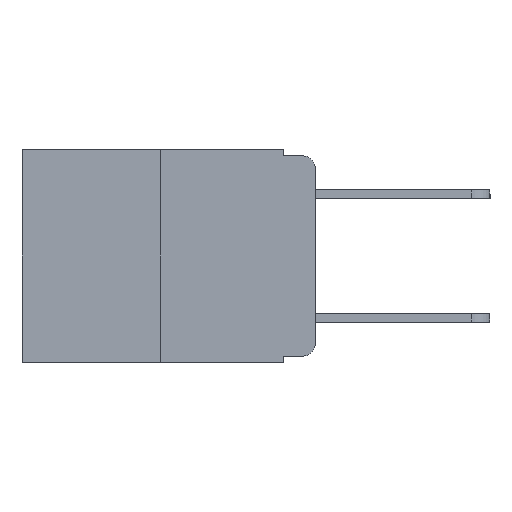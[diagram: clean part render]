
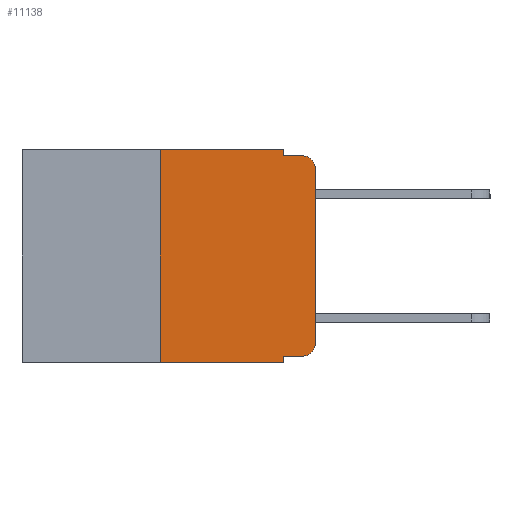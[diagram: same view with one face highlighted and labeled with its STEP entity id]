
A CAD part, left-side view. The second image highlights one B-rep face of the part: STEP entity #11138.
In plain terms, the highlighted planar face has unit normal (-1, 0, 0).
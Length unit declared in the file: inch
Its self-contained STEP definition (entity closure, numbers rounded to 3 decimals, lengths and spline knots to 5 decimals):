
#94 = VERTEX_POINT ( 'NONE', #11074 ) ;
#110 = DIRECTION ( 'NONE',  ( 0., 0., -1. ) ) ;
#378 = LINE ( 'NONE', #8288, #10097 ) ;
#680 = EDGE_CURVE ( 'NONE', #3848, #2437, #4072, .T. ) ;
#988 = VERTEX_POINT ( 'NONE', #6801 ) ;
#1204 = DIRECTION ( 'NONE',  ( 0., -1., 0. ) ) ;
#1396 = LINE ( 'NONE', #10054, #5968 ) ;
#1401 = ORIENTED_EDGE ( 'NONE', *, *, #8843, .F. ) ;
#1557 = VECTOR ( 'NONE', #3485, 39.37008 ) ;
#1706 = CARTESIAN_POINT ( 'NONE',  ( 0., 0.051, 0. ) ) ;
#1749 = ORIENTED_EDGE ( 'NONE', *, *, #1933, .F. ) ;
#1764 = CARTESIAN_POINT ( 'NONE',  ( 0., 0.473, -0.343 ) ) ;
#1769 = CARTESIAN_POINT ( 'NONE',  ( 0., 0.051, 0. ) ) ;
#1846 = EDGE_CURVE ( 'NONE', #5021, #2993, #1396, .T. ) ;
#1866 = EDGE_CURVE ( 'NONE', #2993, #94, #3632, .T. ) ;
#1905 = EDGE_CURVE ( 'NONE', #988, #94, #9902, .T. ) ;
#1933 = EDGE_CURVE ( 'NONE', #4409, #988, #5375, .T. ) ;
#1965 = EDGE_CURVE ( 'NONE', #3848, #10779, #9175, .T. ) ;
#1985 = EDGE_CURVE ( 'NONE', #4274, #2437, #4609, .T. ) ;
#2002 = EDGE_CURVE ( 'NONE', #4274, #9136, #6937, .T. ) ;
#2294 = CARTESIAN_POINT ( 'NONE',  ( 0., 0.473, 0. ) ) ;
#2395 = CARTESIAN_POINT ( 'NONE',  ( 0., 0.02, -0.333 ) ) ;
#2409 = CARTESIAN_POINT ( 'NONE',  ( 0., 0., -0.03 ) ) ;
#2437 = VERTEX_POINT ( 'NONE', #11195 ) ;
#2537 = EDGE_CURVE ( 'NONE', #9136, #5021, #9658, .T. ) ;
#2837 = DIRECTION ( 'NONE',  ( 0., -1., 0. ) ) ;
#2993 = VERTEX_POINT ( 'NONE', #2409 ) ;
#3011 = ORIENTED_EDGE ( 'NONE', *, *, #1866, .T. ) ;
#3067 = CARTESIAN_POINT ( 'NONE',  ( 0., 0.051, 0. ) ) ;
#3081 = ORIENTED_EDGE ( 'NONE', *, *, #1846, .T. ) ;
#3084 = VECTOR ( 'NONE', #1204, 39.37008 ) ;
#3246 = DIRECTION ( 'NONE',  ( 0., 0., -1. ) ) ;
#3353 = ORIENTED_EDGE ( 'NONE', *, *, #2537, .T. ) ;
#3485 = DIRECTION ( 'NONE',  ( 0., -1., 0. ) ) ;
#3632 = CIRCLE ( 'NONE', #4986, 0.02 ) ;
#3761 = AXIS2_PLACEMENT_3D ( 'NONE', #9645, #9270, #9260 ) ;
#3848 = VERTEX_POINT ( 'NONE', #4613 ) ;
#4072 = LINE ( 'NONE', #1764, #1557 ) ;
#4073 = CARTESIAN_POINT ( 'NONE',  ( 0., 0., -0.313 ) ) ;
#4075 = CARTESIAN_POINT ( 'NONE',  ( 0., 0.051, -0.333 ) ) ;
#4274 = VERTEX_POINT ( 'NONE', #9355 ) ;
#4409 = VERTEX_POINT ( 'NONE', #1706 ) ;
#4609 = LINE ( 'NONE', #3067, #8918 ) ;
#4613 = CARTESIAN_POINT ( 'NONE',  ( 0., 0.25, -0.343 ) ) ;
#4986 = AXIS2_PLACEMENT_3D ( 'NONE', #8393, #6985, #7596 ) ;
#5021 = VERTEX_POINT ( 'NONE', #4073 ) ;
#5117 = VECTOR ( 'NONE', #110, 39.37008 ) ;
#5198 = ORIENTED_EDGE ( 'NONE', *, *, #680, .T. ) ;
#5299 = ORIENTED_EDGE ( 'NONE', *, *, #2002, .T. ) ;
#5375 = LINE ( 'NONE', #1769, #5117 ) ;
#5539 = DIRECTION ( 'NONE',  ( 0., -1., 0. ) ) ;
#5758 = ORIENTED_EDGE ( 'NONE', *, *, #1905, .F. ) ;
#5968 = VECTOR ( 'NONE', #10854, 39.37008 ) ;
#6409 = DIRECTION ( 'NONE',  ( 0., 0., 1. ) ) ;
#6436 = EDGE_LOOP ( 'NONE', ( #3081, #3011, #5758, #1749, #1401, #10562, #5198, #8328, #5299, #3353 ) ) ;
#6668 = VECTOR ( 'NONE', #2837, 39.37008 ) ;
#6801 = CARTESIAN_POINT ( 'NONE',  ( 0., 0.051, -0.01 ) ) ;
#6937 = LINE ( 'NONE', #4075, #6668 ) ;
#6985 = DIRECTION ( 'NONE',  ( -1., 0., 0. ) ) ;
#7084 = CARTESIAN_POINT ( 'NONE',  ( 0., 0.051, -0.01 ) ) ;
#7556 = DIRECTION ( 'NONE',  ( 0., 0., -1. ) ) ;
#7596 = DIRECTION ( 'NONE',  ( 0., 0., -1. ) ) ;
#7644 = PLANE ( 'NONE',  #10780 ) ;
#8288 = CARTESIAN_POINT ( 'NONE',  ( 0., 0.473, 0. ) ) ;
#8319 = VECTOR ( 'NONE', #6409, 39.37008 ) ;
#8328 = ORIENTED_EDGE ( 'NONE', *, *, #1985, .F. ) ;
#8393 = CARTESIAN_POINT ( 'NONE',  ( 0., 0.02, -0.03 ) ) ;
#8489 = DIRECTION ( 'NONE',  ( 1., 0., 0. ) ) ;
#8843 = EDGE_CURVE ( 'NONE', #10779, #4409, #378, .T. ) ;
#8918 = VECTOR ( 'NONE', #7556, 39.37008 ) ;
#9136 = VERTEX_POINT ( 'NONE', #2395 ) ;
#9175 = LINE ( 'NONE', #9251, #8319 ) ;
#9251 = CARTESIAN_POINT ( 'NONE',  ( 0., 0.25, 0. ) ) ;
#9260 = DIRECTION ( 'NONE',  ( 0., 0., -1. ) ) ;
#9270 = DIRECTION ( 'NONE',  ( -1., 0., 0. ) ) ;
#9355 = CARTESIAN_POINT ( 'NONE',  ( 0., 0.051, -0.333 ) ) ;
#9645 = CARTESIAN_POINT ( 'NONE',  ( 0., 0.02, -0.313 ) ) ;
#9658 = CIRCLE ( 'NONE', #3761, 0.02 ) ;
#9701 = CARTESIAN_POINT ( 'NONE',  ( 0., 0.25, 0. ) ) ;
#9902 = LINE ( 'NONE', #7084, #3084 ) ;
#10054 = CARTESIAN_POINT ( 'NONE',  ( 0., 0., 0. ) ) ;
#10097 = VECTOR ( 'NONE', #5539, 39.37008 ) ;
#10562 = ORIENTED_EDGE ( 'NONE', *, *, #1965, .F. ) ;
#10771 = FACE_OUTER_BOUND ( 'NONE', #6436, .T. ) ;
#10779 = VERTEX_POINT ( 'NONE', #9701 ) ;
#10780 = AXIS2_PLACEMENT_3D ( 'NONE', #2294, #8489, #3246 ) ;
#10854 = DIRECTION ( 'NONE',  ( 0., 0., 1. ) ) ;
#11074 = CARTESIAN_POINT ( 'NONE',  ( 0., 0.02, -0.01 ) ) ;
#11138 = ADVANCED_FACE ( 'NONE', ( #10771 ), #7644, .F. ) ;
#11195 = CARTESIAN_POINT ( 'NONE',  ( 0., 0.051, -0.343 ) ) ;
